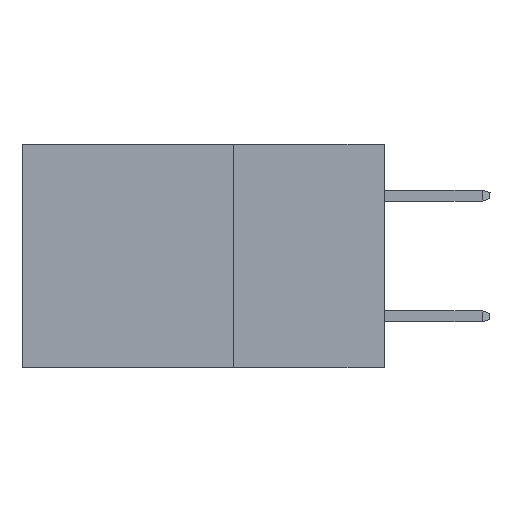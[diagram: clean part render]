
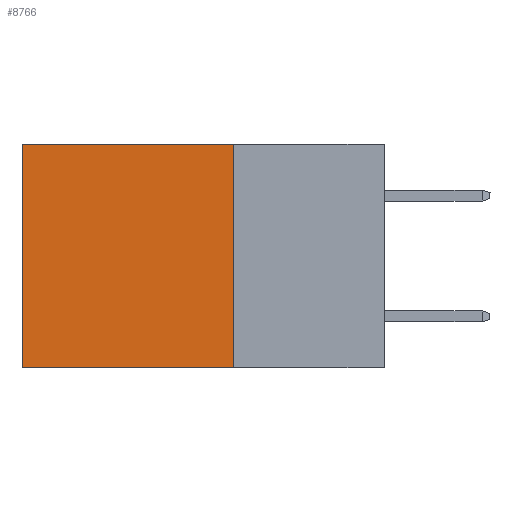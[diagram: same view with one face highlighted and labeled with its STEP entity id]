
A CAD part, left-side view. The second image highlights one B-rep face of the part: STEP entity #8766.
In plain terms, the highlighted planar face has unit normal (-1, 0, 0).
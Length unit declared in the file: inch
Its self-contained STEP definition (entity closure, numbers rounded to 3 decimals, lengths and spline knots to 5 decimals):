
#288 = VERTEX_POINT ( 'NONE', #9679 ) ;
#836 = CARTESIAN_POINT ( 'NONE',  ( 0.298, 0.6, 0. ) ) ;
#1068 = DIRECTION ( 'NONE',  ( 1., 0., 0. ) ) ;
#2907 = VECTOR ( 'NONE', #11829, 39.37008 ) ;
#3215 = LINE ( 'NONE', #14244, #16187 ) ;
#3379 = DIRECTION ( 'NONE',  ( 0., 1., 0. ) ) ;
#5328 = VECTOR ( 'NONE', #9943, 39.37008 ) ;
#5362 = CARTESIAN_POINT ( 'NONE',  ( 0.298, 0.6, 0. ) ) ;
#5526 = CARTESIAN_POINT ( 'NONE',  ( 0.298, 0.25, -0.37 ) ) ;
#6665 = ORIENTED_EDGE ( 'NONE', *, *, #14974, .T. ) ;
#7275 = PLANE ( 'NONE',  #10135 ) ;
#7492 = VECTOR ( 'NONE', #13572, 39.37008 ) ;
#7982 = EDGE_CURVE ( 'NONE', #19628, #288, #11675, .T. ) ;
#8498 = LINE ( 'NONE', #5362, #5328 ) ;
#8766 = ADVANCED_FACE ( 'NONE', ( #20221 ), #7275, .F. ) ;
#9596 = CARTESIAN_POINT ( 'NONE',  ( 0.298, 0.25, 0. ) ) ;
#9679 = CARTESIAN_POINT ( 'NONE',  ( 0.298, 0.25, -0.37 ) ) ;
#9943 = DIRECTION ( 'NONE',  ( 0., 0., -1. ) ) ;
#10135 = AXIS2_PLACEMENT_3D ( 'NONE', #10438, #1068, #11064 ) ;
#10298 = VERTEX_POINT ( 'NONE', #836 ) ;
#10371 = CARTESIAN_POINT ( 'NONE',  ( 0.298, 0.25, 0. ) ) ;
#10438 = CARTESIAN_POINT ( 'NONE',  ( 0.298, 0.25, 0. ) ) ;
#10446 = EDGE_CURVE ( 'NONE', #10298, #11182, #8498, .T. ) ;
#11064 = DIRECTION ( 'NONE',  ( 0., 0., -1. ) ) ;
#11182 = VERTEX_POINT ( 'NONE', #19512 ) ;
#11675 = LINE ( 'NONE', #10371, #7492 ) ;
#11829 = DIRECTION ( 'NONE',  ( 0., 1., 0. ) ) ;
#13572 = DIRECTION ( 'NONE',  ( 0., 0., -1. ) ) ;
#14244 = CARTESIAN_POINT ( 'NONE',  ( 0.298, 0.25, 0. ) ) ;
#14974 = EDGE_CURVE ( 'NONE', #19628, #10298, #3215, .T. ) ;
#15354 = ORIENTED_EDGE ( 'NONE', *, *, #17877, .F. ) ;
#15719 = ORIENTED_EDGE ( 'NONE', *, *, #7982, .F. ) ;
#16187 = VECTOR ( 'NONE', #3379, 39.37008 ) ;
#17877 = EDGE_CURVE ( 'NONE', #288, #11182, #19302, .T. ) ;
#18653 = ORIENTED_EDGE ( 'NONE', *, *, #10446, .T. ) ;
#19112 = EDGE_LOOP ( 'NONE', ( #18653, #15354, #15719, #6665 ) ) ;
#19302 = LINE ( 'NONE', #5526, #2907 ) ;
#19512 = CARTESIAN_POINT ( 'NONE',  ( 0.298, 0.6, -0.37 ) ) ;
#19628 = VERTEX_POINT ( 'NONE', #9596 ) ;
#20221 = FACE_OUTER_BOUND ( 'NONE', #19112, .T. ) ;
